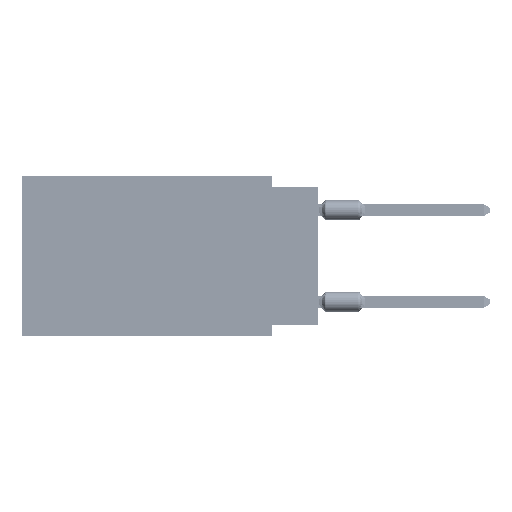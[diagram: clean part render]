
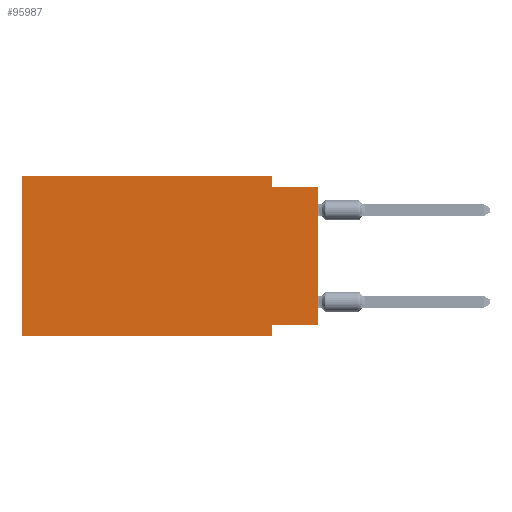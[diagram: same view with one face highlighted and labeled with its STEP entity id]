
A CAD part, left-side view. The second image highlights one B-rep face of the part: STEP entity #95987.
In plain terms, the highlighted planar face has unit normal (-1, 0, 0).
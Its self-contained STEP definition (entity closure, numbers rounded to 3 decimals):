
#2736 = CARTESIAN_POINT ( 'NONE',  ( 0., 16.383, 0. ) ) ;
#2827 = CARTESIAN_POINT ( 'NONE',  ( 0., 0., 0. ) ) ;
#3638 = LINE ( 'NONE', #52170, #81779 ) ;
#8282 = VECTOR ( 'NONE', #60118, 1000. ) ;
#9924 = VERTEX_POINT ( 'NONE', #98422 ) ;
#10379 = CARTESIAN_POINT ( 'NONE',  ( 0., 2.54, 0. ) ) ;
#10800 = VECTOR ( 'NONE', #50895, 1000. ) ;
#10839 = EDGE_CURVE ( 'NONE', #66750, #14556, #50575, .T. ) ;
#13926 = LINE ( 'NONE', #100572, #71510 ) ;
#14556 = VERTEX_POINT ( 'NONE', #10379 ) ;
#16440 = AXIS2_PLACEMENT_3D ( 'NONE', #77212, #37568, #54222 ) ;
#17060 = CARTESIAN_POINT ( 'NONE',  ( 0., 2.54, -8.255 ) ) ;
#17404 = CARTESIAN_POINT ( 'NONE',  ( 0., 16.383, -8.89 ) ) ;
#18803 = DIRECTION ( 'NONE',  ( 0., 0., -1. ) ) ;
#19564 = CARTESIAN_POINT ( 'NONE',  ( 0., 2.54, 0. ) ) ;
#20463 = LINE ( 'NONE', #2736, #8282 ) ;
#21061 = VERTEX_POINT ( 'NONE', #63483 ) ;
#23322 = ORIENTED_EDGE ( 'NONE', *, *, #87065, .F. ) ;
#25854 = ORIENTED_EDGE ( 'NONE', *, *, #10839, .F. ) ;
#31207 = DIRECTION ( 'NONE',  ( 0., 1., 0. ) ) ;
#31334 = ORIENTED_EDGE ( 'NONE', *, *, #74615, .F. ) ;
#31846 = EDGE_CURVE ( 'NONE', #9924, #44584, #90525, .T. ) ;
#35942 = CARTESIAN_POINT ( 'NONE',  ( 0., 16.383, 0. ) ) ;
#37568 = DIRECTION ( 'NONE',  ( 1., 0., 0. ) ) ;
#38519 = CARTESIAN_POINT ( 'NONE',  ( 0., 0., -8.255 ) ) ;
#38688 = VERTEX_POINT ( 'NONE', #17404 ) ;
#41000 = ORIENTED_EDGE ( 'NONE', *, *, #80517, .F. ) ;
#41121 = VECTOR ( 'NONE', #31207, 1000. ) ;
#42361 = EDGE_CURVE ( 'NONE', #14556, #79692, #74902, .T. ) ;
#43859 = ORIENTED_EDGE ( 'NONE', *, *, #42361, .F. ) ;
#44191 = CARTESIAN_POINT ( 'NONE',  ( 0., 0., -0.635 ) ) ;
#44584 = VERTEX_POINT ( 'NONE', #44191 ) ;
#45325 = VECTOR ( 'NONE', #82402, 1000. ) ;
#50575 = LINE ( 'NONE', #35942, #45325 ) ;
#50895 = DIRECTION ( 'NONE',  ( 0., 0., -1. ) ) ;
#51904 = CARTESIAN_POINT ( 'NONE',  ( 0., 2.54, -0.635 ) ) ;
#52170 = CARTESIAN_POINT ( 'NONE',  ( 0., 2.54, -8.89 ) ) ;
#54222 = DIRECTION ( 'NONE',  ( 0., 0., -1. ) ) ;
#56553 = VECTOR ( 'NONE', #62041, 1000. ) ;
#57459 = ORIENTED_EDGE ( 'NONE', *, *, #96277, .T. ) ;
#60118 = DIRECTION ( 'NONE',  ( 0., 0., 1. ) ) ;
#61404 = DIRECTION ( 'NONE',  ( 0., -1., 0. ) ) ;
#62041 = DIRECTION ( 'NONE',  ( 0., -1., 0. ) ) ;
#62044 = PLANE ( 'NONE',  #16440 ) ;
#62851 = ORIENTED_EDGE ( 'NONE', *, *, #87692, .F. ) ;
#63483 = CARTESIAN_POINT ( 'NONE',  ( 0., 2.54, -8.89 ) ) ;
#66515 = DIRECTION ( 'NONE',  ( 0., 0., 1. ) ) ;
#66750 = VERTEX_POINT ( 'NONE', #91880 ) ;
#69996 = VECTOR ( 'NONE', #66515, 1000. ) ;
#71510 = VECTOR ( 'NONE', #61404, 1000. ) ;
#74615 = EDGE_CURVE ( 'NONE', #9924, #74649, #96395, .T. ) ;
#74649 = VERTEX_POINT ( 'NONE', #17060 ) ;
#74902 = LINE ( 'NONE', #19564, #10800 ) ;
#76173 = LINE ( 'NONE', #92340, #56553 ) ;
#77212 = CARTESIAN_POINT ( 'NONE',  ( 0., 16.383, 0. ) ) ;
#79692 = VERTEX_POINT ( 'NONE', #51904 ) ;
#80517 = EDGE_CURVE ( 'NONE', #74649, #21061, #3638, .T. ) ;
#81779 = VECTOR ( 'NONE', #18803, 1000. ) ;
#82402 = DIRECTION ( 'NONE',  ( 0., -1., 0. ) ) ;
#84426 = EDGE_LOOP ( 'NONE', ( #97396, #23322, #43859, #25854, #62851, #57459, #41000, #31334 ) ) ;
#87065 = EDGE_CURVE ( 'NONE', #79692, #44584, #76173, .T. ) ;
#87692 = EDGE_CURVE ( 'NONE', #38688, #66750, #20463, .T. ) ;
#90525 = LINE ( 'NONE', #2827, #69996 ) ;
#91880 = CARTESIAN_POINT ( 'NONE',  ( 0., 16.383, 0. ) ) ;
#92340 = CARTESIAN_POINT ( 'NONE',  ( 0., 0., -0.635 ) ) ;
#93374 = FACE_OUTER_BOUND ( 'NONE', #84426, .T. ) ;
#95987 = ADVANCED_FACE ( 'NONE', ( #93374 ), #62044, .F. ) ;
#96277 = EDGE_CURVE ( 'NONE', #38688, #21061, #13926, .T. ) ;
#96395 = LINE ( 'NONE', #38519, #41121 ) ;
#97396 = ORIENTED_EDGE ( 'NONE', *, *, #31846, .T. ) ;
#98422 = CARTESIAN_POINT ( 'NONE',  ( 0., 0., -8.255 ) ) ;
#100572 = CARTESIAN_POINT ( 'NONE',  ( 0., 16.383, -8.89 ) ) ;
